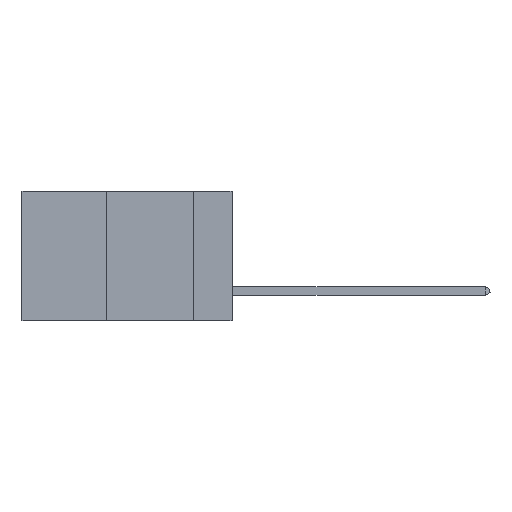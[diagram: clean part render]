
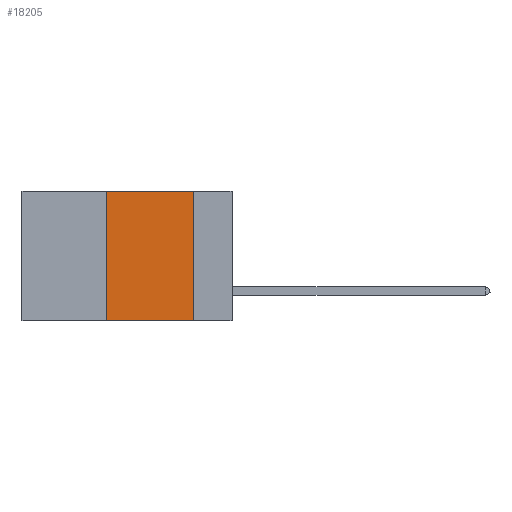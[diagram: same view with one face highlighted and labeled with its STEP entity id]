
A CAD part, left-side view. The second image highlights one B-rep face of the part: STEP entity #18205.
In plain terms, the highlighted planar face has unit normal (-1, 0, 0).
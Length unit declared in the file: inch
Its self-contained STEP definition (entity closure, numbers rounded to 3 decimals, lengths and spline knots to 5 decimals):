
#104 = PLANE ( 'NONE',  #23614 ) ;
#203 = CARTESIAN_POINT ( 'NONE',  ( 0., 0.6, 0. ) ) ;
#511 = ORIENTED_EDGE ( 'NONE', *, *, #3920, .F. ) ;
#1792 = ORIENTED_EDGE ( 'NONE', *, *, #10484, .F. ) ;
#2388 = DIRECTION ( 'NONE',  ( 0., 0., -1. ) ) ;
#2535 = DIRECTION ( 'NONE',  ( 0., 0., -1. ) ) ;
#2597 = DIRECTION ( 'NONE',  ( 0., -1., 0. ) ) ;
#3146 = CARTESIAN_POINT ( 'NONE',  ( 0., 0.36, 0. ) ) ;
#3920 = EDGE_CURVE ( 'NONE', #22549, #9146, #21599, .T. ) ;
#4777 = DIRECTION ( 'NONE',  ( 0., -1., 0. ) ) ;
#4976 = CARTESIAN_POINT ( 'NONE',  ( 0., 0.11, -0.37 ) ) ;
#6326 = VECTOR ( 'NONE', #2597, 39.37008 ) ;
#9146 = VERTEX_POINT ( 'NONE', #13356 ) ;
#10484 = EDGE_CURVE ( 'NONE', #9146, #26954, #12494, .T. ) ;
#10796 = CARTESIAN_POINT ( 'NONE',  ( 0., 0.36, 0. ) ) ;
#10887 = DIRECTION ( 'NONE',  ( 0., 0., 1. ) ) ;
#11175 = CARTESIAN_POINT ( 'NONE',  ( 0., 0.11, 0. ) ) ;
#11652 = CARTESIAN_POINT ( 'NONE',  ( 0., 0.6, 0. ) ) ;
#11730 = VERTEX_POINT ( 'NONE', #26845 ) ;
#12494 = LINE ( 'NONE', #11175, #18900 ) ;
#13002 = ORIENTED_EDGE ( 'NONE', *, *, #18785, .T. ) ;
#13356 = CARTESIAN_POINT ( 'NONE',  ( 0., 0.11, 0. ) ) ;
#15363 = DIRECTION ( 'NONE',  ( 1., 0., 0. ) ) ;
#16265 = EDGE_LOOP ( 'NONE', ( #1792, #511, #23234, #13002 ) ) ;
#17482 = FACE_OUTER_BOUND ( 'NONE', #16265, .T. ) ;
#17889 = VECTOR ( 'NONE', #4777, 39.37008 ) ;
#17893 = CARTESIAN_POINT ( 'NONE',  ( 0., 0.6, -0.37 ) ) ;
#18205 = ADVANCED_FACE ( 'NONE', ( #17482 ), #104, .F. ) ;
#18785 = EDGE_CURVE ( 'NONE', #11730, #26954, #27291, .T. ) ;
#18900 = VECTOR ( 'NONE', #2535, 39.37008 ) ;
#21599 = LINE ( 'NONE', #11652, #17889 ) ;
#22189 = EDGE_CURVE ( 'NONE', #11730, #22549, #26984, .T. ) ;
#22549 = VERTEX_POINT ( 'NONE', #3146 ) ;
#23234 = ORIENTED_EDGE ( 'NONE', *, *, #22189, .F. ) ;
#23614 = AXIS2_PLACEMENT_3D ( 'NONE', #203, #15363, #2388 ) ;
#24244 = VECTOR ( 'NONE', #10887, 39.37008 ) ;
#26845 = CARTESIAN_POINT ( 'NONE',  ( 0., 0.36, -0.37 ) ) ;
#26954 = VERTEX_POINT ( 'NONE', #4976 ) ;
#26984 = LINE ( 'NONE', #10796, #24244 ) ;
#27291 = LINE ( 'NONE', #17893, #6326 ) ;
